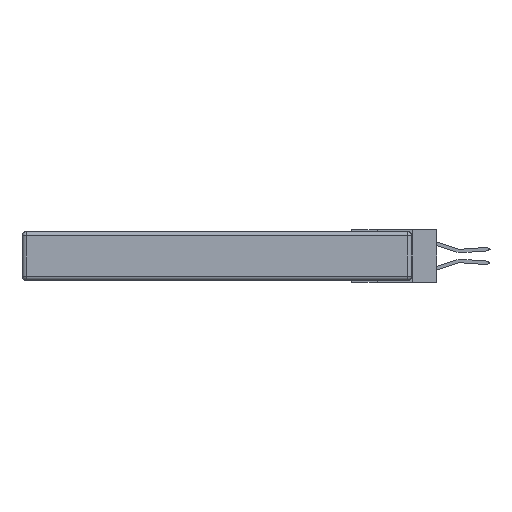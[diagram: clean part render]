
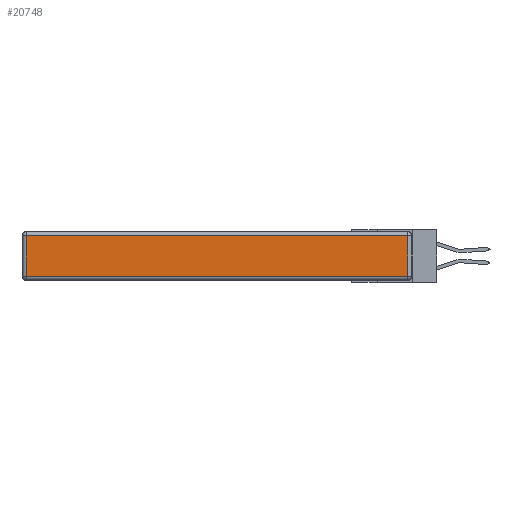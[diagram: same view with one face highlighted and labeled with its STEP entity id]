
A CAD part, left-side view. The second image highlights one B-rep face of the part: STEP entity #20748.
In plain terms, the highlighted planar face has unit normal (-1, 0, 0).
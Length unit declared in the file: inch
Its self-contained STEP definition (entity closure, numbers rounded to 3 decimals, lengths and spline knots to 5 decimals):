
#1030 = LINE ( 'NONE', #6048, #15855 ) ;
#1143 = DIRECTION ( 'NONE',  ( 0., 1., 0. ) ) ;
#1516 = CARTESIAN_POINT ( 'NONE',  ( 0., 2.72, -0.313 ) ) ;
#2823 = EDGE_CURVE ( 'NONE', #27107, #15227, #6237, .T. ) ;
#3369 = CARTESIAN_POINT ( 'NONE',  ( 0., 2.72, -0.343 ) ) ;
#4175 = FACE_OUTER_BOUND ( 'NONE', #25796, .T. ) ;
#4559 = VERTEX_POINT ( 'NONE', #20512 ) ;
#5589 = VECTOR ( 'NONE', #19110, 39.37008 ) ;
#5895 = DIRECTION ( 'NONE',  ( 0., 0., -1. ) ) ;
#6048 = CARTESIAN_POINT ( 'NONE',  ( 0., 2.75, -0.03 ) ) ;
#6237 = LINE ( 'NONE', #13048, #32024 ) ;
#8760 = CARTESIAN_POINT ( 'NONE',  ( 0., 0.03, -0.03 ) ) ;
#10145 = ORIENTED_EDGE ( 'NONE', *, *, #26618, .T. ) ;
#10197 = VECTOR ( 'NONE', #5895, 39.37008 ) ;
#13048 = CARTESIAN_POINT ( 'NONE',  ( 0., 0., -0.313 ) ) ;
#13807 = ORIENTED_EDGE ( 'NONE', *, *, #2823, .T. ) ;
#14628 = EDGE_CURVE ( 'NONE', #4559, #27107, #21085, .T. ) ;
#15227 = VERTEX_POINT ( 'NONE', #24248 ) ;
#15516 = DIRECTION ( 'NONE',  ( 0., -1., 0. ) ) ;
#15855 = VECTOR ( 'NONE', #1143, 39.37008 ) ;
#17704 = AXIS2_PLACEMENT_3D ( 'NONE', #24442, #21612, #26736 ) ;
#18629 = ORIENTED_EDGE ( 'NONE', *, *, #14628, .T. ) ;
#19110 = DIRECTION ( 'NONE',  ( 0., 0., 1. ) ) ;
#20512 = CARTESIAN_POINT ( 'NONE',  ( 0., 2.72, -0.03 ) ) ;
#20748 = ADVANCED_FACE ( 'NONE', ( #4175 ), #24229, .T. ) ;
#21085 = LINE ( 'NONE', #3369, #10197 ) ;
#21317 = EDGE_CURVE ( 'NONE', #22231, #4559, #1030, .T. ) ;
#21384 = ORIENTED_EDGE ( 'NONE', *, *, #21317, .T. ) ;
#21612 = DIRECTION ( 'NONE',  ( -1., 0., 0. ) ) ;
#22231 = VERTEX_POINT ( 'NONE', #8760 ) ;
#24229 = PLANE ( 'NONE',  #17704 ) ;
#24248 = CARTESIAN_POINT ( 'NONE',  ( 0., 0.03, -0.313 ) ) ;
#24442 = CARTESIAN_POINT ( 'NONE',  ( 0., 0., -0.343 ) ) ;
#25796 = EDGE_LOOP ( 'NONE', ( #13807, #10145, #21384, #18629 ) ) ;
#26618 = EDGE_CURVE ( 'NONE', #15227, #22231, #30597, .T. ) ;
#26736 = DIRECTION ( 'NONE',  ( 0., 0., 1. ) ) ;
#27107 = VERTEX_POINT ( 'NONE', #1516 ) ;
#28965 = CARTESIAN_POINT ( 'NONE',  ( 0., 0.03, -0.343 ) ) ;
#30597 = LINE ( 'NONE', #28965, #5589 ) ;
#32024 = VECTOR ( 'NONE', #15516, 39.37008 ) ;
